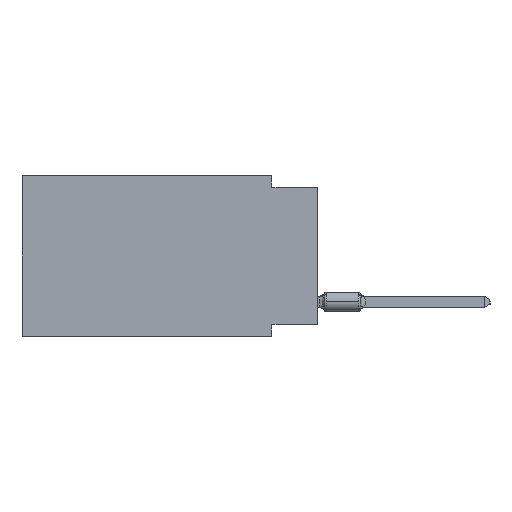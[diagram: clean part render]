
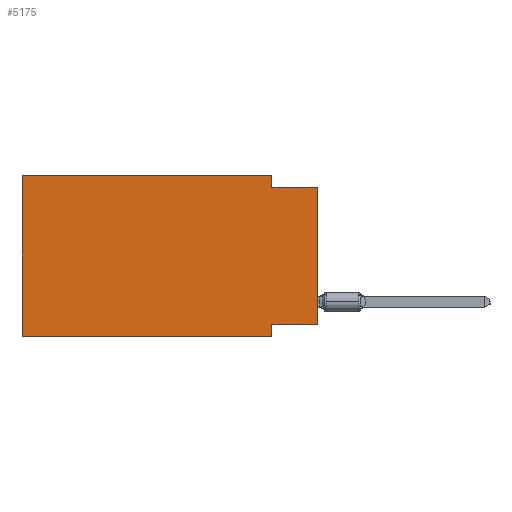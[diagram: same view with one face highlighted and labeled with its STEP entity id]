
A CAD part, left-side view. The second image highlights one B-rep face of the part: STEP entity #5175.
In plain terms, the highlighted planar face has unit normal (-1, 0, 0).
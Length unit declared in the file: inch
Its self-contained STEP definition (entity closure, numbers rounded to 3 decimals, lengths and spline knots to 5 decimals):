
#291 = EDGE_LOOP ( 'NONE', ( #55587, #24206, #33229, #48904, #53268, #30091, #7369, #36161 ) ) ;
#1865 = CARTESIAN_POINT ( 'NONE',  ( 0., 0.645, 0. ) ) ;
#3944 = DIRECTION ( 'NONE',  ( 0., 0., -1. ) ) ;
#4874 = VECTOR ( 'NONE', #19362, 39.37008 ) ;
#5175 = ADVANCED_FACE ( 'NONE', ( #19371 ), #42358, .F. ) ;
#7369 = ORIENTED_EDGE ( 'NONE', *, *, #31520, .F. ) ;
#7561 = CARTESIAN_POINT ( 'NONE',  ( 0., 0., -0.025 ) ) ;
#9080 = LINE ( 'NONE', #30636, #54105 ) ;
#9633 = CARTESIAN_POINT ( 'NONE',  ( 0., 0., -0.025 ) ) ;
#11287 = DIRECTION ( 'NONE',  ( 0., -1., 0. ) ) ;
#11430 = CARTESIAN_POINT ( 'NONE',  ( 0., 0.1, -0.325 ) ) ;
#13033 = VERTEX_POINT ( 'NONE', #7561 ) ;
#14011 = VERTEX_POINT ( 'NONE', #22162 ) ;
#14122 = CARTESIAN_POINT ( 'NONE',  ( 0., 0.1, -0.35 ) ) ;
#14220 = CARTESIAN_POINT ( 'NONE',  ( 0., 0.1, -0.025 ) ) ;
#14231 = VECTOR ( 'NONE', #55691, 39.37008 ) ;
#17357 = DIRECTION ( 'NONE',  ( 0., 0., 1. ) ) ;
#19202 = EDGE_CURVE ( 'NONE', #22460, #13033, #29558, .T. ) ;
#19362 = DIRECTION ( 'NONE',  ( 0., -1., 0. ) ) ;
#19371 = FACE_OUTER_BOUND ( 'NONE', #291, .T. ) ;
#19540 = CARTESIAN_POINT ( 'NONE',  ( 0., 0.645, -0.35 ) ) ;
#20434 = LINE ( 'NONE', #1865, #27563 ) ;
#22162 = CARTESIAN_POINT ( 'NONE',  ( 0., 0., -0.325 ) ) ;
#22460 = VERTEX_POINT ( 'NONE', #14220 ) ;
#23420 = LINE ( 'NONE', #46137, #30624 ) ;
#24206 = ORIENTED_EDGE ( 'NONE', *, *, #19202, .F. ) ;
#25259 = VECTOR ( 'NONE', #3944, 39.37008 ) ;
#25672 = EDGE_CURVE ( 'NONE', #46496, #22460, #53201, .T. ) ;
#27563 = VECTOR ( 'NONE', #11287, 39.37008 ) ;
#28939 = CARTESIAN_POINT ( 'NONE',  ( 0., 0.645, 0. ) ) ;
#29558 = LINE ( 'NONE', #9633, #4874 ) ;
#29736 = VERTEX_POINT ( 'NONE', #28939 ) ;
#30091 = ORIENTED_EDGE ( 'NONE', *, *, #37898, .T. ) ;
#30624 = VECTOR ( 'NONE', #40852, 39.37008 ) ;
#30636 = CARTESIAN_POINT ( 'NONE',  ( 0., 0., 0. ) ) ;
#30785 = CARTESIAN_POINT ( 'NONE',  ( 0., 0.1, 0. ) ) ;
#30875 = EDGE_CURVE ( 'NONE', #14011, #13033, #9080, .T. ) ;
#31520 = EDGE_CURVE ( 'NONE', #36625, #34899, #23420, .T. ) ;
#32186 = AXIS2_PLACEMENT_3D ( 'NONE', #50915, #50632, #37639 ) ;
#33229 = ORIENTED_EDGE ( 'NONE', *, *, #25672, .F. ) ;
#33275 = CARTESIAN_POINT ( 'NONE',  ( 0., 0.645, -0.35 ) ) ;
#34899 = VERTEX_POINT ( 'NONE', #14122 ) ;
#36161 = ORIENTED_EDGE ( 'NONE', *, *, #36407, .F. ) ;
#36407 = EDGE_CURVE ( 'NONE', #14011, #36625, #39234, .T. ) ;
#36625 = VERTEX_POINT ( 'NONE', #11430 ) ;
#36695 = CARTESIAN_POINT ( 'NONE',  ( 0., 0.1, 0. ) ) ;
#37639 = DIRECTION ( 'NONE',  ( 0., 0., -1. ) ) ;
#37898 = EDGE_CURVE ( 'NONE', #45760, #34899, #46846, .T. ) ;
#39234 = LINE ( 'NONE', #57241, #53819 ) ;
#39580 = EDGE_CURVE ( 'NONE', #29736, #46496, #20434, .T. ) ;
#40852 = DIRECTION ( 'NONE',  ( 0., 0., -1. ) ) ;
#42358 = PLANE ( 'NONE',  #32186 ) ;
#42524 = CARTESIAN_POINT ( 'NONE',  ( 0., 0.645, 0. ) ) ;
#45760 = VERTEX_POINT ( 'NONE', #19540 ) ;
#46137 = CARTESIAN_POINT ( 'NONE',  ( 0., 0.1, -0.35 ) ) ;
#46496 = VERTEX_POINT ( 'NONE', #36695 ) ;
#46846 = LINE ( 'NONE', #33275, #14231 ) ;
#48358 = DIRECTION ( 'NONE',  ( 0., 1., 0. ) ) ;
#48904 = ORIENTED_EDGE ( 'NONE', *, *, #39580, .F. ) ;
#50273 = VECTOR ( 'NONE', #56126, 39.37008 ) ;
#50632 = DIRECTION ( 'NONE',  ( 1., 0., 0. ) ) ;
#50915 = CARTESIAN_POINT ( 'NONE',  ( 0., 0.645, 0. ) ) ;
#51118 = EDGE_CURVE ( 'NONE', #45760, #29736, #56687, .T. ) ;
#53201 = LINE ( 'NONE', #30785, #25259 ) ;
#53268 = ORIENTED_EDGE ( 'NONE', *, *, #51118, .F. ) ;
#53819 = VECTOR ( 'NONE', #48358, 39.37008 ) ;
#54105 = VECTOR ( 'NONE', #17357, 39.37008 ) ;
#55587 = ORIENTED_EDGE ( 'NONE', *, *, #30875, .T. ) ;
#55691 = DIRECTION ( 'NONE',  ( 0., -1., 0. ) ) ;
#56126 = DIRECTION ( 'NONE',  ( 0., 0., 1. ) ) ;
#56687 = LINE ( 'NONE', #42524, #50273 ) ;
#57241 = CARTESIAN_POINT ( 'NONE',  ( 0., 0., -0.325 ) ) ;
